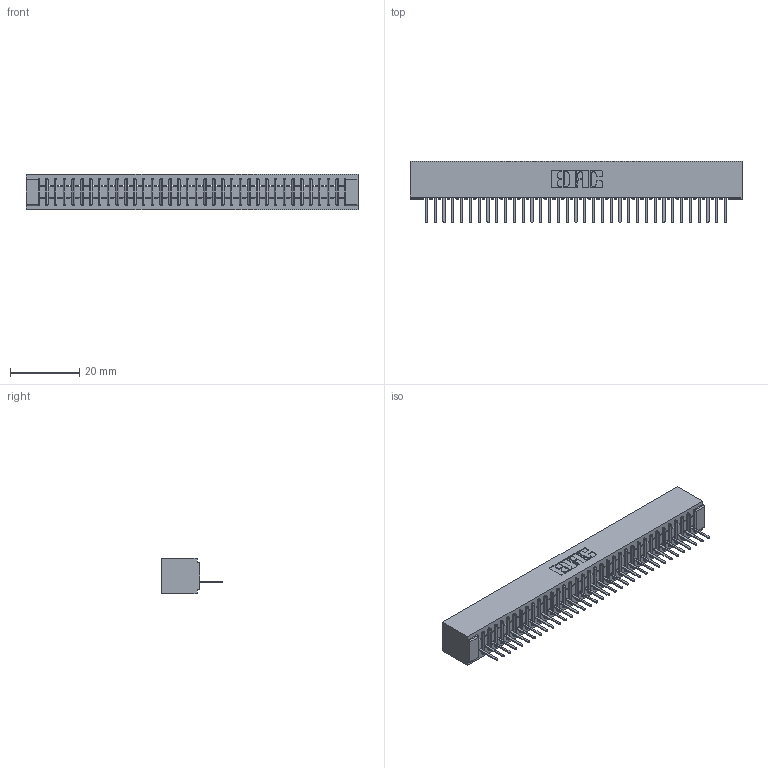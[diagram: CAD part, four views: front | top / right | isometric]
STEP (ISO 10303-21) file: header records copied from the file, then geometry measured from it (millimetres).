
FILE_DESCRIPTION (( 'STEP AP203' ), '1' );
FILE_NAME ('391-035-521-101.STEP', '2018-08-08T23:06:17', ( '' ), ( '' ), 'SwSTEP 2.0', 'SolidWorks 2016', '' );
FILE_SCHEMA (( 'CONFIG_CONTROL_DESIGN' ));
Length unit declared in the file: inch
Products named in the file (3): 341 Part_No Mounting Lugs; 341-292-001_341-292-121; 391-035-521-101
Assembly tree (36 placements, depth 2):
  391-035-521-101
    341 Part_No Mounting Lugs
    341-292-001_341-292-121  x35
Bounding box: 95.89 x 17.7 x 10.16 mm (x, y, z)
Volume: 7086.4 mm3; surface area: 11431.7 mm2
Topology: 36 solids, 36 shells, 2978 faces, 8587 edges, 5510 vertices
Faces by surface type: plane 1849, cylinder 989, sphere 72, torus 68
Entity records: 41892 total; most frequent: CARTESIAN_POINT 7114, ORIENTED_EDGE 7102, DIRECTION 6871, EDGE_CURVE 3551, LINE 2865, VECTOR 2865, VERTEX_POINT 2246, AXIS2_PLACEMENT_3D 2003
